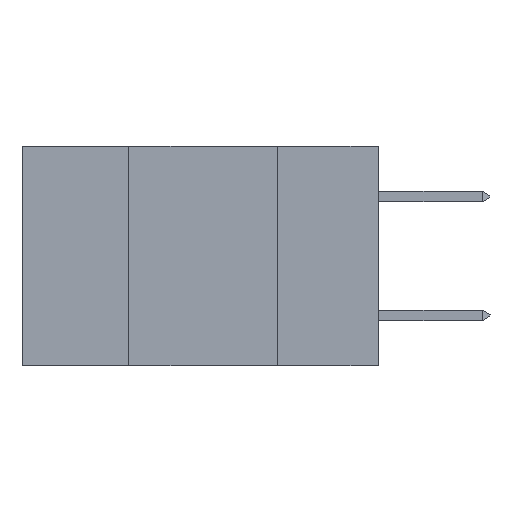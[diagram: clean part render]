
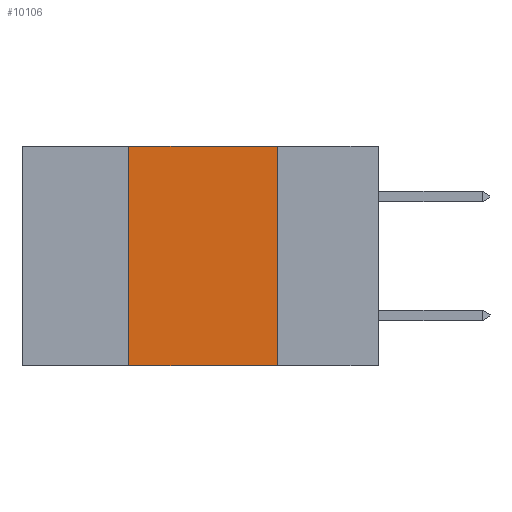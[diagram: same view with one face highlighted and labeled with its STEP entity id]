
A CAD part, left-side view. The second image highlights one B-rep face of the part: STEP entity #10106.
In plain terms, the highlighted planar face has unit normal (-1, 0, 0).
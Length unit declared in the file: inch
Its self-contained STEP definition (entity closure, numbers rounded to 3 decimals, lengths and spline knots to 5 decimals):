
#256 = EDGE_LOOP ( 'NONE', ( #5148, #1076, #7893, #4526 ) ) ;
#1076 = ORIENTED_EDGE ( 'NONE', *, *, #6768, .F. ) ;
#1846 = CARTESIAN_POINT ( 'NONE',  ( 0., 0.6, -0.37 ) ) ;
#2557 = AXIS2_PLACEMENT_3D ( 'NONE', #8795, #3342, #6039 ) ;
#2941 = EDGE_CURVE ( 'NONE', #5502, #3889, #5873, .T. ) ;
#3342 = DIRECTION ( 'NONE',  ( 1., 0., 0. ) ) ;
#3348 = FACE_OUTER_BOUND ( 'NONE', #256, .T. ) ;
#3494 = CARTESIAN_POINT ( 'NONE',  ( 0., 0.17, -0.37 ) ) ;
#3599 = LINE ( 'NONE', #7034, #6835 ) ;
#3889 = VERTEX_POINT ( 'NONE', #10594 ) ;
#4276 = PLANE ( 'NONE',  #2557 ) ;
#4526 = ORIENTED_EDGE ( 'NONE', *, *, #2941, .T. ) ;
#5148 = ORIENTED_EDGE ( 'NONE', *, *, #10472, .F. ) ;
#5255 = VERTEX_POINT ( 'NONE', #8875 ) ;
#5270 = LINE ( 'NONE', #3494, #6131 ) ;
#5502 = VERTEX_POINT ( 'NONE', #5503 ) ;
#5503 = CARTESIAN_POINT ( 'NONE',  ( 0., 0.42, -0.37 ) ) ;
#5573 = VECTOR ( 'NONE', #8881, 39.37008 ) ;
#5873 = LINE ( 'NONE', #1846, #8534 ) ;
#6039 = DIRECTION ( 'NONE',  ( 0., 0., -1. ) ) ;
#6131 = VECTOR ( 'NONE', #8002, 39.37008 ) ;
#6768 = EDGE_CURVE ( 'NONE', #5255, #8782, #7984, .T. ) ;
#6835 = VECTOR ( 'NONE', #7937, 39.37008 ) ;
#7034 = CARTESIAN_POINT ( 'NONE',  ( 0., 0.42, -0.37 ) ) ;
#7893 = ORIENTED_EDGE ( 'NONE', *, *, #10468, .F. ) ;
#7937 = DIRECTION ( 'NONE',  ( 0., 0., 1. ) ) ;
#7964 = CARTESIAN_POINT ( 'NONE',  ( 0., 0.6, 0. ) ) ;
#7984 = LINE ( 'NONE', #7964, #5573 ) ;
#8002 = DIRECTION ( 'NONE',  ( 0., 0., -1. ) ) ;
#8534 = VECTOR ( 'NONE', #11100, 39.37008 ) ;
#8746 = CARTESIAN_POINT ( 'NONE',  ( 0., 0.17, 0. ) ) ;
#8782 = VERTEX_POINT ( 'NONE', #8746 ) ;
#8795 = CARTESIAN_POINT ( 'NONE',  ( 0., 0.6, 0. ) ) ;
#8875 = CARTESIAN_POINT ( 'NONE',  ( 0., 0.42, 0. ) ) ;
#8881 = DIRECTION ( 'NONE',  ( 0., -1., 0. ) ) ;
#10106 = ADVANCED_FACE ( 'NONE', ( #3348 ), #4276, .F. ) ;
#10468 = EDGE_CURVE ( 'NONE', #5502, #5255, #3599, .T. ) ;
#10472 = EDGE_CURVE ( 'NONE', #8782, #3889, #5270, .T. ) ;
#10594 = CARTESIAN_POINT ( 'NONE',  ( 0., 0.17, -0.37 ) ) ;
#11100 = DIRECTION ( 'NONE',  ( 0., -1., 0. ) ) ;
